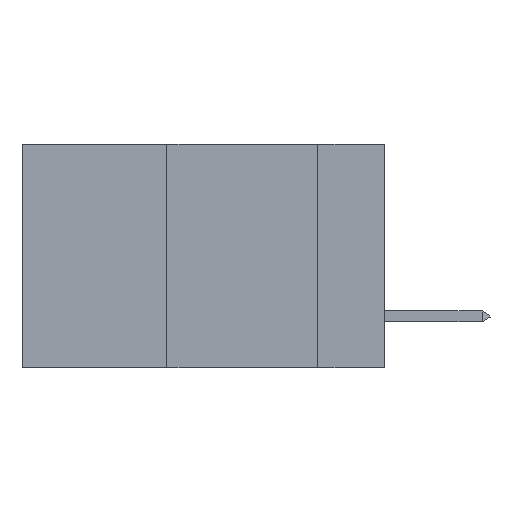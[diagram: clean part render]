
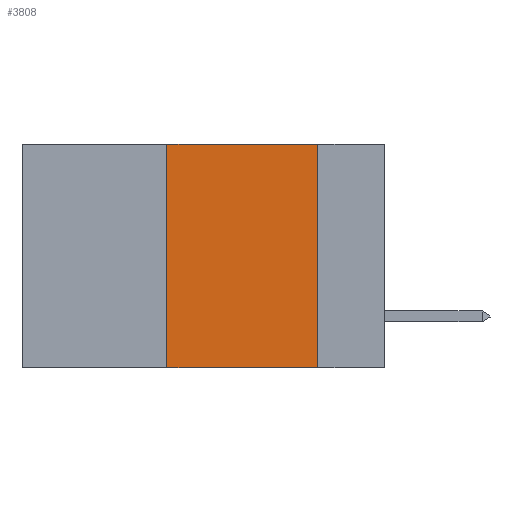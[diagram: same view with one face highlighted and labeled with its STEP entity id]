
A CAD part, left-side view. The second image highlights one B-rep face of the part: STEP entity #3808.
In plain terms, the highlighted planar face has unit normal (-1, 0, 0).
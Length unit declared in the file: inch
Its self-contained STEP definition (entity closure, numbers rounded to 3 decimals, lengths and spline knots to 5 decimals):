
#631 = CARTESIAN_POINT ( 'NONE',  ( 0., 0.6, -0.37 ) ) ;
#979 = DIRECTION ( 'NONE',  ( 0., -1., 0. ) ) ;
#3036 = LINE ( 'NONE', #5486, #11825 ) ;
#3366 = DIRECTION ( 'NONE',  ( 0., -1., 0. ) ) ;
#3725 = VERTEX_POINT ( 'NONE', #5308 ) ;
#3808 = ADVANCED_FACE ( 'NONE', ( #13514 ), #8440, .F. ) ;
#4352 = VERTEX_POINT ( 'NONE', #5993 ) ;
#4471 = ORIENTED_EDGE ( 'NONE', *, *, #21650, .F. ) ;
#5308 = CARTESIAN_POINT ( 'NONE',  ( 0., 0.36, -0.37 ) ) ;
#5400 = CARTESIAN_POINT ( 'NONE',  ( 0., 0.36, 0. ) ) ;
#5486 = CARTESIAN_POINT ( 'NONE',  ( 0., 0.11, 0. ) ) ;
#5993 = CARTESIAN_POINT ( 'NONE',  ( 0., 0.11, 0. ) ) ;
#6857 = ORIENTED_EDGE ( 'NONE', *, *, #14632, .F. ) ;
#8397 = DIRECTION ( 'NONE',  ( 0., 0., -1. ) ) ;
#8440 = PLANE ( 'NONE',  #21325 ) ;
#10983 = VECTOR ( 'NONE', #17723, 39.37008 ) ;
#11028 = CARTESIAN_POINT ( 'NONE',  ( 0., 0.36, 0. ) ) ;
#11664 = LINE ( 'NONE', #29996, #30117 ) ;
#11825 = VECTOR ( 'NONE', #22542, 39.37008 ) ;
#12950 = ORIENTED_EDGE ( 'NONE', *, *, #16816, .T. ) ;
#13514 = FACE_OUTER_BOUND ( 'NONE', #23068, .T. ) ;
#14632 = EDGE_CURVE ( 'NONE', #3725, #16480, #24198, .T. ) ;
#16480 = VERTEX_POINT ( 'NONE', #11028 ) ;
#16816 = EDGE_CURVE ( 'NONE', #3725, #17289, #25908, .T. ) ;
#17289 = VERTEX_POINT ( 'NONE', #26910 ) ;
#17568 = VECTOR ( 'NONE', #979, 39.37008 ) ;
#17723 = DIRECTION ( 'NONE',  ( 0., 0., 1. ) ) ;
#18648 = EDGE_CURVE ( 'NONE', #4352, #17289, #3036, .T. ) ;
#21325 = AXIS2_PLACEMENT_3D ( 'NONE', #27993, #26098, #8397 ) ;
#21650 = EDGE_CURVE ( 'NONE', #16480, #4352, #11664, .T. ) ;
#22542 = DIRECTION ( 'NONE',  ( 0., 0., -1. ) ) ;
#23068 = EDGE_LOOP ( 'NONE', ( #28398, #4471, #6857, #12950 ) ) ;
#24198 = LINE ( 'NONE', #5400, #10983 ) ;
#25908 = LINE ( 'NONE', #631, #17568 ) ;
#26098 = DIRECTION ( 'NONE',  ( 1., 0., 0. ) ) ;
#26910 = CARTESIAN_POINT ( 'NONE',  ( 0., 0.11, -0.37 ) ) ;
#27993 = CARTESIAN_POINT ( 'NONE',  ( 0., 0.6, 0. ) ) ;
#28398 = ORIENTED_EDGE ( 'NONE', *, *, #18648, .F. ) ;
#29996 = CARTESIAN_POINT ( 'NONE',  ( 0., 0.6, 0. ) ) ;
#30117 = VECTOR ( 'NONE', #3366, 39.37008 ) ;
